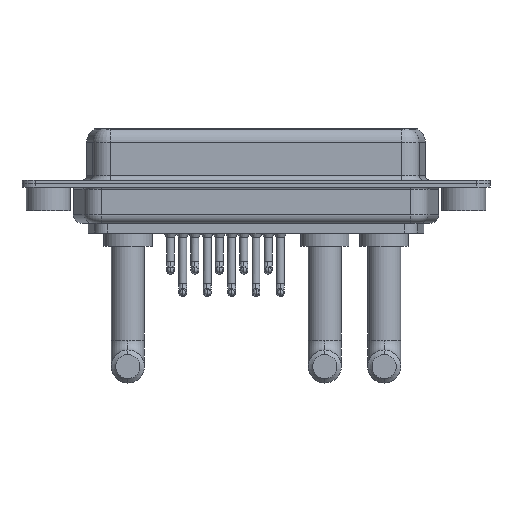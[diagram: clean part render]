
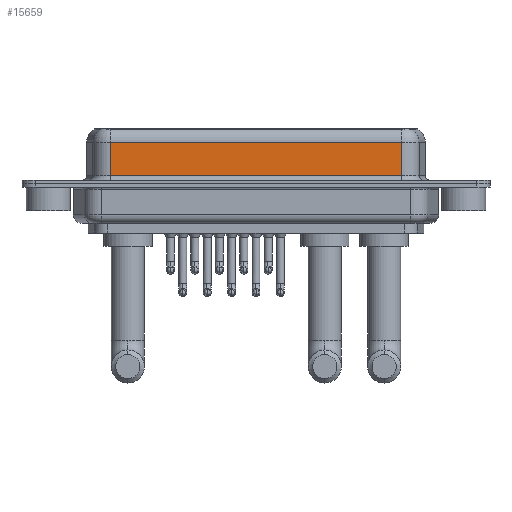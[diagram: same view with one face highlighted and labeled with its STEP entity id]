
A CAD part, front view. The second image highlights one B-rep face of the part: STEP entity #15659.
In plain terms, the highlighted planar face has unit normal (0, -1, 0).
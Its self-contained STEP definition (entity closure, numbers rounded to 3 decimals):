
#406 = EDGE_CURVE ( 'NONE', #7325, #8038, #9215, .T. ) ;
#520 = CARTESIAN_POINT ( 'NONE',  ( 7.013, -3.95, 4.65 ) ) ;
#1577 = LINE ( 'NONE', #6117, #7401 ) ;
#1678 = AXIS2_PLACEMENT_3D ( 'NONE', #3817, #15622, #2383 ) ;
#2138 = EDGE_LOOP ( 'NONE', ( #17140, #8078, #10110, #18636 ) ) ;
#2383 = DIRECTION ( 'NONE',  ( 0., 0., 1. ) ) ;
#2902 = VERTEX_POINT ( 'NONE', #520 ) ;
#3192 = CARTESIAN_POINT ( 'NONE',  ( 40.037, -3.95, 6.4 ) ) ;
#3447 = DIRECTION ( 'NONE',  ( 1., 0., 0. ) ) ;
#3498 = CARTESIAN_POINT ( 'NONE',  ( 7.013, -3.95, 6.4 ) ) ;
#3817 = CARTESIAN_POINT ( 'NONE',  ( 40.037, -3.95, 6.4 ) ) ;
#5276 = PLANE ( 'NONE',  #1678 ) ;
#6117 = CARTESIAN_POINT ( 'NONE',  ( 40.037, -3.95, 4.65 ) ) ;
#7012 = VECTOR ( 'NONE', #9136, 1000. ) ;
#7109 = EDGE_CURVE ( 'NONE', #7325, #2902, #1577, .T. ) ;
#7325 = VERTEX_POINT ( 'NONE', #9305 ) ;
#7401 = VECTOR ( 'NONE', #14928, 1000. ) ;
#7658 = LINE ( 'NONE', #16708, #17162 ) ;
#8038 = VERTEX_POINT ( 'NONE', #8960 ) ;
#8078 = ORIENTED_EDGE ( 'NONE', *, *, #7109, .T. ) ;
#8367 = VECTOR ( 'NONE', #18109, 1000. ) ;
#8960 = CARTESIAN_POINT ( 'NONE',  ( 40.037, -3.95, 0.9 ) ) ;
#9136 = DIRECTION ( 'NONE',  ( 0., 0., -1. ) ) ;
#9215 = LINE ( 'NONE', #3192, #8367 ) ;
#9305 = CARTESIAN_POINT ( 'NONE',  ( 40.037, -3.95, 4.65 ) ) ;
#10110 = ORIENTED_EDGE ( 'NONE', *, *, #18376, .T. ) ;
#10383 = VERTEX_POINT ( 'NONE', #13277 ) ;
#13277 = CARTESIAN_POINT ( 'NONE',  ( 7.013, -3.95, 0.9 ) ) ;
#13494 = LINE ( 'NONE', #3498, #7012 ) ;
#14928 = DIRECTION ( 'NONE',  ( -1., 0., 0. ) ) ;
#15622 = DIRECTION ( 'NONE',  ( 0., 1., 0. ) ) ;
#15659 = ADVANCED_FACE ( 'NONE', ( #18522 ), #5276, .F. ) ;
#16173 = EDGE_CURVE ( 'NONE', #10383, #8038, #7658, .T. ) ;
#16708 = CARTESIAN_POINT ( 'NONE',  ( 40.037, -3.95, 0.9 ) ) ;
#17140 = ORIENTED_EDGE ( 'NONE', *, *, #406, .F. ) ;
#17162 = VECTOR ( 'NONE', #3447, 1000. ) ;
#18109 = DIRECTION ( 'NONE',  ( 0., 0., -1. ) ) ;
#18376 = EDGE_CURVE ( 'NONE', #2902, #10383, #13494, .T. ) ;
#18522 = FACE_OUTER_BOUND ( 'NONE', #2138, .T. ) ;
#18636 = ORIENTED_EDGE ( 'NONE', *, *, #16173, .T. ) ;
